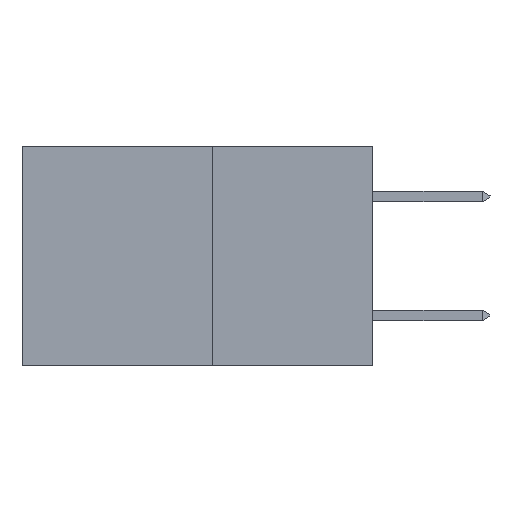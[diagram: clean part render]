
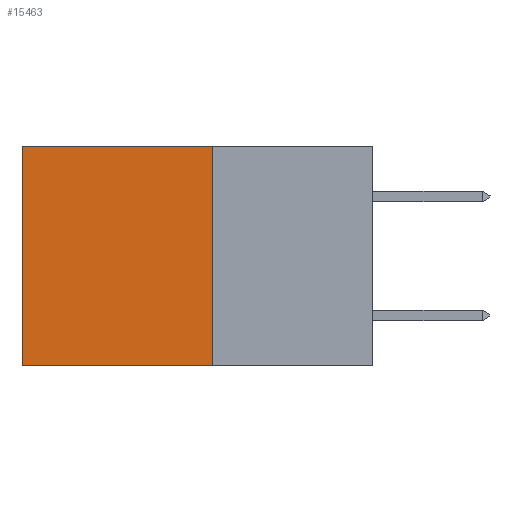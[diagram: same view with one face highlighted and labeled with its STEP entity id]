
A CAD part, left-side view. The second image highlights one B-rep face of the part: STEP entity #15463.
In plain terms, the highlighted planar face has unit normal (-1, 0, 0).
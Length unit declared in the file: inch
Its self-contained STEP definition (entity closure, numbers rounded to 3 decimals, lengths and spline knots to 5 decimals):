
#128 = LINE ( 'NONE', #9787, #10243 ) ;
#298 = CARTESIAN_POINT ( 'NONE',  ( 0.277, 0.59, 0. ) ) ;
#1300 = EDGE_LOOP ( 'NONE', ( #2965, #9956, #8865, #15093 ) ) ;
#1375 = AXIS2_PLACEMENT_3D ( 'NONE', #5750, #3177, #11752 ) ;
#1978 = EDGE_CURVE ( 'NONE', #14438, #6377, #11914, .T. ) ;
#2331 = LINE ( 'NONE', #8726, #14865 ) ;
#2965 = ORIENTED_EDGE ( 'NONE', *, *, #15118, .T. ) ;
#2998 = EDGE_CURVE ( 'NONE', #14438, #10458, #11521, .T. ) ;
#3177 = DIRECTION ( 'NONE',  ( 1., 0., 0. ) ) ;
#3676 = CARTESIAN_POINT ( 'NONE',  ( 0.277, 0.27, -0.37 ) ) ;
#3788 = CARTESIAN_POINT ( 'NONE',  ( 0.277, 0.27, 0. ) ) ;
#4272 = VERTEX_POINT ( 'NONE', #8378 ) ;
#4928 = DIRECTION ( 'NONE',  ( 0., 1., 0. ) ) ;
#5142 = DIRECTION ( 'NONE',  ( 0., 0., -1. ) ) ;
#5201 = DIRECTION ( 'NONE',  ( 0., 0., -1. ) ) ;
#5566 = VECTOR ( 'NONE', #5201, 39.37008 ) ;
#5750 = CARTESIAN_POINT ( 'NONE',  ( 0.277, 0.27, -0.37 ) ) ;
#6377 = VERTEX_POINT ( 'NONE', #9944 ) ;
#8378 = CARTESIAN_POINT ( 'NONE',  ( 0.277, 0.59, -0.37 ) ) ;
#8726 = CARTESIAN_POINT ( 'NONE',  ( 0.277, 0.59, -0.37 ) ) ;
#8865 = ORIENTED_EDGE ( 'NONE', *, *, #1978, .F. ) ;
#9593 = CARTESIAN_POINT ( 'NONE',  ( 0.277, 0.27, 0. ) ) ;
#9787 = CARTESIAN_POINT ( 'NONE',  ( 0.277, 0.27, -0.37 ) ) ;
#9944 = CARTESIAN_POINT ( 'NONE',  ( 0.277, 0.27, -0.37 ) ) ;
#9956 = ORIENTED_EDGE ( 'NONE', *, *, #10781, .F. ) ;
#10243 = VECTOR ( 'NONE', #4928, 39.37008 ) ;
#10458 = VERTEX_POINT ( 'NONE', #298 ) ;
#10565 = PLANE ( 'NONE',  #1375 ) ;
#10781 = EDGE_CURVE ( 'NONE', #6377, #4272, #128, .T. ) ;
#11521 = LINE ( 'NONE', #9593, #14236 ) ;
#11752 = DIRECTION ( 'NONE',  ( 0., 0., -1. ) ) ;
#11914 = LINE ( 'NONE', #3676, #5566 ) ;
#12280 = DIRECTION ( 'NONE',  ( 0., 1., 0. ) ) ;
#13587 = FACE_OUTER_BOUND ( 'NONE', #1300, .T. ) ;
#14236 = VECTOR ( 'NONE', #12280, 39.37008 ) ;
#14438 = VERTEX_POINT ( 'NONE', #3788 ) ;
#14865 = VECTOR ( 'NONE', #5142, 39.37008 ) ;
#15093 = ORIENTED_EDGE ( 'NONE', *, *, #2998, .T. ) ;
#15118 = EDGE_CURVE ( 'NONE', #10458, #4272, #2331, .T. ) ;
#15463 = ADVANCED_FACE ( 'NONE', ( #13587 ), #10565, .F. ) ;
